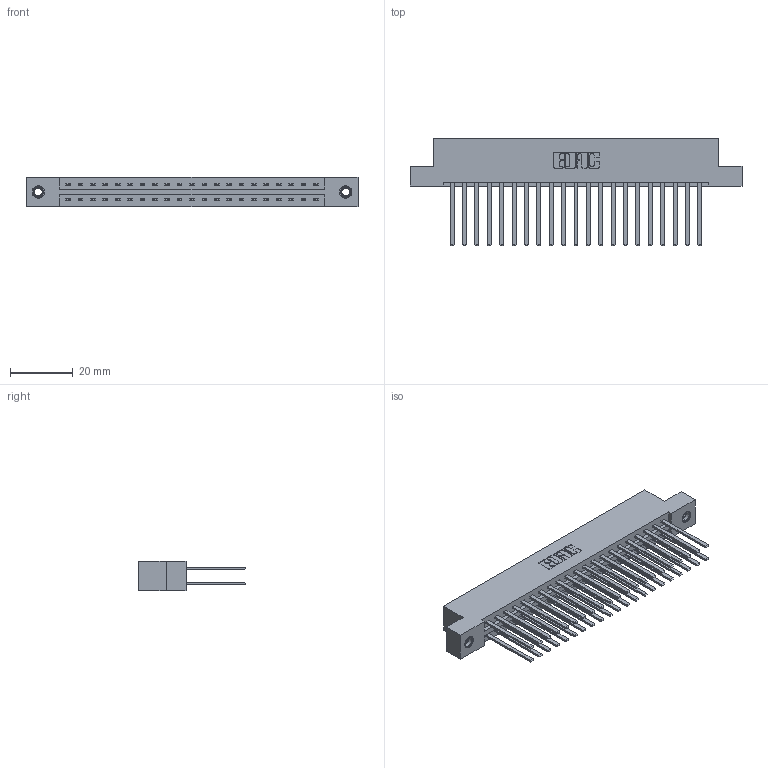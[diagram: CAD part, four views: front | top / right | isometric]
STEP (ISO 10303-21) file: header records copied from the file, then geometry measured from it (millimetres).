
FILE_DESCRIPTION (( 'STEP AP203' ), '1' );
FILE_NAME ('337-042-544-207.STEP', '2019-10-09T12:24:07', ( '' ), ( '' ), 'SwSTEP 2.0', 'SolidWorks 2016', '' );
FILE_SCHEMA (( 'CONFIG_CONTROL_DESIGN' ));
Length unit declared in the file: inch
Products named in the file (4): 337-042-544-207; 337 Part_Flush Mounting Lugs - 0.156 Dia-TI; 345-250-001_345-250-005-103; 345-292-001_345-293-144
Assembly tree (45 placements, depth 2):
  337-042-544-207
    337 Part_Flush Mounting Lugs - 0.156 Dia-TI
    345-292-001_345-293-144  x42
    345-250-001_345-250-005-103  x2
Bounding box: 106.22 x 34.3 x 9.4 mm (x, y, z)
Volume: 11490.3 mm3; surface area: 14745.1 mm2
Topology: 45 solids, 45 shells, 2190 faces, 6453 edges, 4238 vertices
Faces by surface type: plane 1530, cylinder 644, cone 12, torus 4
Entity records: 20000 total; most frequent: CARTESIAN_POINT 3365, ORIENTED_EDGE 3294, DIRECTION 2929, EDGE_CURVE 1647, LINE 1503, VECTOR 1503, VERTEX_POINT 1092, AXIS2_PLACEMENT_3D 713
